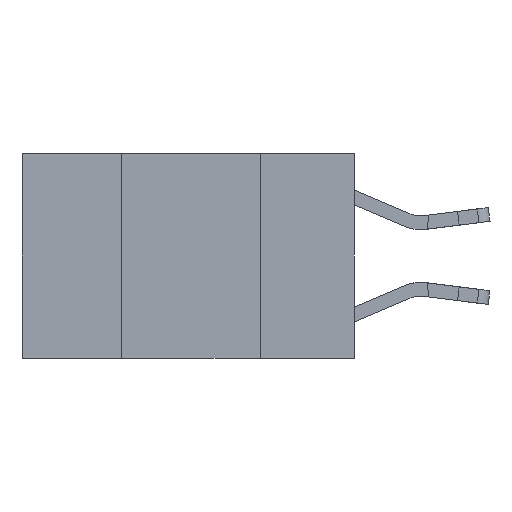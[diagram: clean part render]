
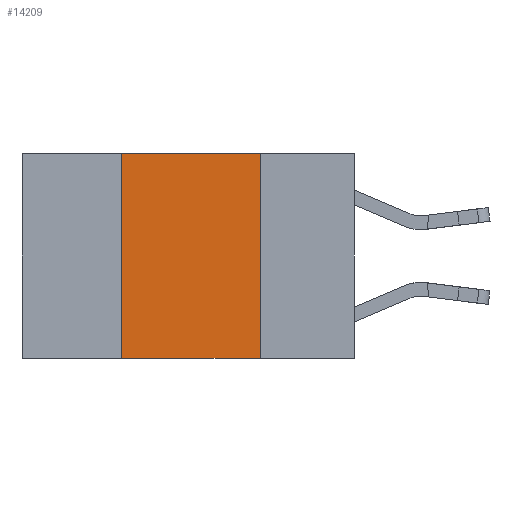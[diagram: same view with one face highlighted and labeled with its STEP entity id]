
A CAD part, left-side view. The second image highlights one B-rep face of the part: STEP entity #14209.
In plain terms, the highlighted planar face has unit normal (-1, 0, 0).
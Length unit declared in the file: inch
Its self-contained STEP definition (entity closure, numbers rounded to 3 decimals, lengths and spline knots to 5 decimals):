
#218 = VERTEX_POINT ( 'NONE', #8741 ) ;
#262 = DIRECTION ( 'NONE',  ( 1., 0., 0. ) ) ;
#384 = EDGE_CURVE ( 'NONE', #8513, #7346, #512, .T. ) ;
#512 = LINE ( 'NONE', #14220, #13858 ) ;
#688 = CARTESIAN_POINT ( 'NONE',  ( 0., 0.42, 0. ) ) ;
#1357 = DIRECTION ( 'NONE',  ( 0., 0., 1. ) ) ;
#1895 = LINE ( 'NONE', #14964, #11792 ) ;
#2849 = EDGE_CURVE ( 'NONE', #218, #4423, #1895, .T. ) ;
#3530 = DIRECTION ( 'NONE',  ( 0., -1., 0. ) ) ;
#3736 = EDGE_CURVE ( 'NONE', #218, #8513, #5747, .T. ) ;
#3741 = ORIENTED_EDGE ( 'NONE', *, *, #384, .F. ) ;
#4423 = VERTEX_POINT ( 'NONE', #14156 ) ;
#4592 = EDGE_CURVE ( 'NONE', #7346, #4423, #7162, .T. ) ;
#5747 = LINE ( 'NONE', #6636, #15089 ) ;
#5976 = EDGE_LOOP ( 'NONE', ( #14384, #3741, #10595, #11432 ) ) ;
#6636 = CARTESIAN_POINT ( 'NONE',  ( 0., 0.42, 0. ) ) ;
#7162 = LINE ( 'NONE', #9366, #7570 ) ;
#7346 = VERTEX_POINT ( 'NONE', #12469 ) ;
#7570 = VECTOR ( 'NONE', #10659, 39.37008 ) ;
#7771 = AXIS2_PLACEMENT_3D ( 'NONE', #10610, #262, #9371 ) ;
#8148 = FACE_OUTER_BOUND ( 'NONE', #5976, .T. ) ;
#8513 = VERTEX_POINT ( 'NONE', #688 ) ;
#8741 = CARTESIAN_POINT ( 'NONE',  ( 0., 0.42, -0.37 ) ) ;
#9366 = CARTESIAN_POINT ( 'NONE',  ( 0., 0.17, 0. ) ) ;
#9371 = DIRECTION ( 'NONE',  ( 0., 0., -1. ) ) ;
#10595 = ORIENTED_EDGE ( 'NONE', *, *, #3736, .F. ) ;
#10610 = CARTESIAN_POINT ( 'NONE',  ( 0., 0.6, 0. ) ) ;
#10659 = DIRECTION ( 'NONE',  ( 0., 0., -1. ) ) ;
#11432 = ORIENTED_EDGE ( 'NONE', *, *, #2849, .T. ) ;
#11792 = VECTOR ( 'NONE', #3530, 39.37008 ) ;
#12469 = CARTESIAN_POINT ( 'NONE',  ( 0., 0.17, 0. ) ) ;
#13858 = VECTOR ( 'NONE', #15592, 39.37008 ) ;
#14156 = CARTESIAN_POINT ( 'NONE',  ( 0., 0.17, -0.37 ) ) ;
#14209 = ADVANCED_FACE ( 'NONE', ( #8148 ), #14435, .F. ) ;
#14220 = CARTESIAN_POINT ( 'NONE',  ( 0., 0.6, 0. ) ) ;
#14384 = ORIENTED_EDGE ( 'NONE', *, *, #4592, .F. ) ;
#14435 = PLANE ( 'NONE',  #7771 ) ;
#14964 = CARTESIAN_POINT ( 'NONE',  ( 0., 0.6, -0.37 ) ) ;
#15089 = VECTOR ( 'NONE', #1357, 39.37008 ) ;
#15592 = DIRECTION ( 'NONE',  ( 0., -1., 0. ) ) ;
